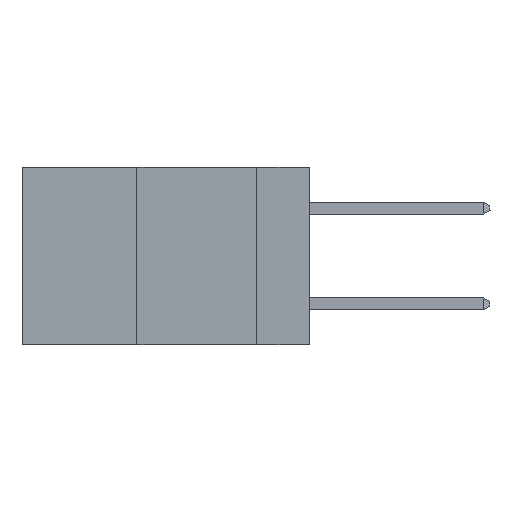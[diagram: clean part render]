
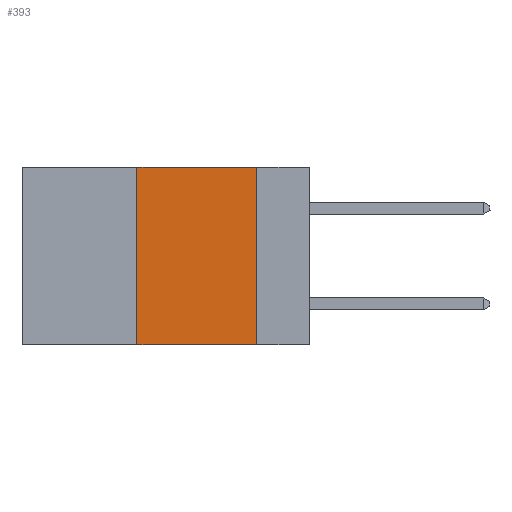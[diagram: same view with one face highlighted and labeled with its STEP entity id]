
A CAD part, left-side view. The second image highlights one B-rep face of the part: STEP entity #393.
In plain terms, the highlighted planar face has unit normal (-1, 0, 0).
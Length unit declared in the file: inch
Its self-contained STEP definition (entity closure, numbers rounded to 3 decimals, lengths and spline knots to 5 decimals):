
#393 = ADVANCED_FACE ( 'NONE', ( #11598 ), #18462, .F. ) ;
#642 = DIRECTION ( 'NONE',  ( 0., -1., 0. ) ) ;
#838 = CARTESIAN_POINT ( 'NONE',  ( 0., 0.6, 0. ) ) ;
#1478 = EDGE_CURVE ( 'NONE', #2334, #24728, #9404, .T. ) ;
#1933 = LINE ( 'NONE', #2887, #19723 ) ;
#2334 = VERTEX_POINT ( 'NONE', #25178 ) ;
#2503 = VERTEX_POINT ( 'NONE', #8025 ) ;
#2681 = DIRECTION ( 'NONE',  ( 0., 0., -1. ) ) ;
#2727 = ORIENTED_EDGE ( 'NONE', *, *, #7812, .F. ) ;
#2775 = DIRECTION ( 'NONE',  ( 0., 0., -1. ) ) ;
#2887 = CARTESIAN_POINT ( 'NONE',  ( 0., 0.6, -0.37 ) ) ;
#4822 = CARTESIAN_POINT ( 'NONE',  ( 0., 0.6, 0. ) ) ;
#4943 = DIRECTION ( 'NONE',  ( 1., 0., 0. ) ) ;
#6664 = VECTOR ( 'NONE', #2775, 39.37008 ) ;
#6986 = CARTESIAN_POINT ( 'NONE',  ( 0., 0.36, 0. ) ) ;
#7812 = EDGE_CURVE ( 'NONE', #9305, #2503, #18964, .T. ) ;
#8025 = CARTESIAN_POINT ( 'NONE',  ( 0., 0.36, 0. ) ) ;
#8604 = EDGE_LOOP ( 'NONE', ( #9164, #15225, #2727, #12592 ) ) ;
#8752 = EDGE_CURVE ( 'NONE', #9305, #24728, #1933, .T. ) ;
#9164 = ORIENTED_EDGE ( 'NONE', *, *, #1478, .F. ) ;
#9305 = VERTEX_POINT ( 'NONE', #17036 ) ;
#9404 = LINE ( 'NONE', #14250, #6664 ) ;
#10569 = LINE ( 'NONE', #4822, #16982 ) ;
#11598 = FACE_OUTER_BOUND ( 'NONE', #8604, .T. ) ;
#12592 = ORIENTED_EDGE ( 'NONE', *, *, #8752, .T. ) ;
#14250 = CARTESIAN_POINT ( 'NONE',  ( 0., 0.11, 0. ) ) ;
#15225 = ORIENTED_EDGE ( 'NONE', *, *, #21287, .F. ) ;
#15399 = AXIS2_PLACEMENT_3D ( 'NONE', #838, #4943, #2681 ) ;
#15686 = CARTESIAN_POINT ( 'NONE',  ( 0., 0.11, -0.37 ) ) ;
#16982 = VECTOR ( 'NONE', #642, 39.37008 ) ;
#17036 = CARTESIAN_POINT ( 'NONE',  ( 0., 0.36, -0.37 ) ) ;
#18462 = PLANE ( 'NONE',  #15399 ) ;
#18799 = DIRECTION ( 'NONE',  ( 0., 0., 1. ) ) ;
#18964 = LINE ( 'NONE', #6986, #20817 ) ;
#19723 = VECTOR ( 'NONE', #22456, 39.37008 ) ;
#20817 = VECTOR ( 'NONE', #18799, 39.37008 ) ;
#21287 = EDGE_CURVE ( 'NONE', #2503, #2334, #10569, .T. ) ;
#22456 = DIRECTION ( 'NONE',  ( 0., -1., 0. ) ) ;
#24728 = VERTEX_POINT ( 'NONE', #15686 ) ;
#25178 = CARTESIAN_POINT ( 'NONE',  ( 0., 0.11, 0. ) ) ;
